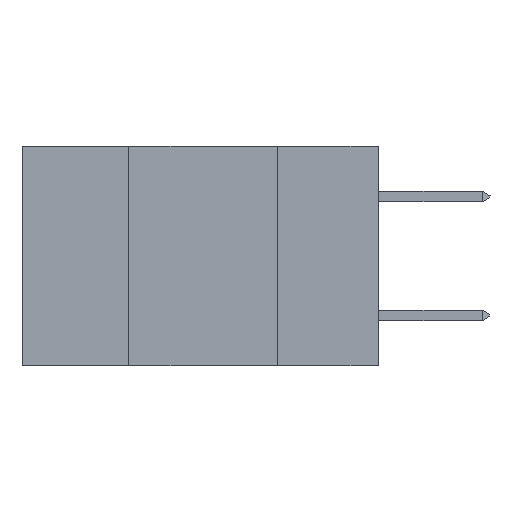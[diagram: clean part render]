
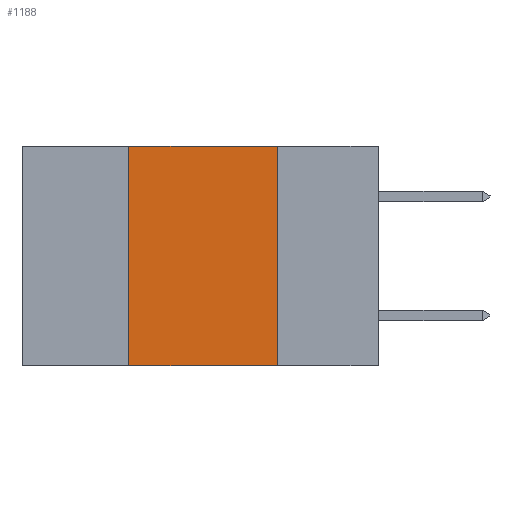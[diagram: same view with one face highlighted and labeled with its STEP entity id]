
A CAD part, left-side view. The second image highlights one B-rep face of the part: STEP entity #1188.
In plain terms, the highlighted planar face has unit normal (-1, 0, 0).
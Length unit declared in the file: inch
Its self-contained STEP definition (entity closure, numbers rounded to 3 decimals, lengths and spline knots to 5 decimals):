
#215 = DIRECTION ( 'NONE',  ( 0., -1., 0. ) ) ;
#390 = DIRECTION ( 'NONE',  ( 0., 0., 1. ) ) ;
#531 = VECTOR ( 'NONE', #12730, 39.37008 ) ;
#797 = DIRECTION ( 'NONE',  ( 0., 0., -1. ) ) ;
#866 = EDGE_LOOP ( 'NONE', ( #4749, #6793, #9677, #8339 ) ) ;
#991 = CARTESIAN_POINT ( 'NONE',  ( 0., 0.42, -0.37 ) ) ;
#1188 = ADVANCED_FACE ( 'NONE', ( #12073 ), #7169, .F. ) ;
#1453 = EDGE_CURVE ( 'NONE', #10099, #10242, #7891, .T. ) ;
#1494 = VECTOR ( 'NONE', #215, 39.37008 ) ;
#2509 = CARTESIAN_POINT ( 'NONE',  ( 0., 0.6, -0.37 ) ) ;
#2744 = LINE ( 'NONE', #2509, #1494 ) ;
#2998 = DIRECTION ( 'NONE',  ( 0., -1., 0. ) ) ;
#3047 = EDGE_CURVE ( 'NONE', #11562, #15285, #2744, .T. ) ;
#4749 = ORIENTED_EDGE ( 'NONE', *, *, #6866, .F. ) ;
#5438 = LINE ( 'NONE', #7657, #531 ) ;
#6793 = ORIENTED_EDGE ( 'NONE', *, *, #1453, .F. ) ;
#6866 = EDGE_CURVE ( 'NONE', #10242, #15285, #5438, .T. ) ;
#6915 = EDGE_CURVE ( 'NONE', #11562, #10099, #9116, .T. ) ;
#7169 = PLANE ( 'NONE',  #9157 ) ;
#7657 = CARTESIAN_POINT ( 'NONE',  ( 0., 0.17, -0.37 ) ) ;
#7891 = LINE ( 'NONE', #10257, #10480 ) ;
#7935 = CARTESIAN_POINT ( 'NONE',  ( 0., 0.42, 0. ) ) ;
#8339 = ORIENTED_EDGE ( 'NONE', *, *, #3047, .T. ) ;
#9116 = LINE ( 'NONE', #12887, #10956 ) ;
#9157 = AXIS2_PLACEMENT_3D ( 'NONE', #11988, #16090, #797 ) ;
#9677 = ORIENTED_EDGE ( 'NONE', *, *, #6915, .F. ) ;
#10099 = VERTEX_POINT ( 'NONE', #7935 ) ;
#10242 = VERTEX_POINT ( 'NONE', #11108 ) ;
#10257 = CARTESIAN_POINT ( 'NONE',  ( 0., 0.6, 0. ) ) ;
#10480 = VECTOR ( 'NONE', #2998, 39.37008 ) ;
#10956 = VECTOR ( 'NONE', #390, 39.37008 ) ;
#11108 = CARTESIAN_POINT ( 'NONE',  ( 0., 0.17, 0. ) ) ;
#11244 = CARTESIAN_POINT ( 'NONE',  ( 0., 0.17, -0.37 ) ) ;
#11562 = VERTEX_POINT ( 'NONE', #991 ) ;
#11988 = CARTESIAN_POINT ( 'NONE',  ( 0., 0.6, 0. ) ) ;
#12073 = FACE_OUTER_BOUND ( 'NONE', #866, .T. ) ;
#12730 = DIRECTION ( 'NONE',  ( 0., 0., -1. ) ) ;
#12887 = CARTESIAN_POINT ( 'NONE',  ( 0., 0.42, -0.37 ) ) ;
#15285 = VERTEX_POINT ( 'NONE', #11244 ) ;
#16090 = DIRECTION ( 'NONE',  ( 1., 0., 0. ) ) ;
